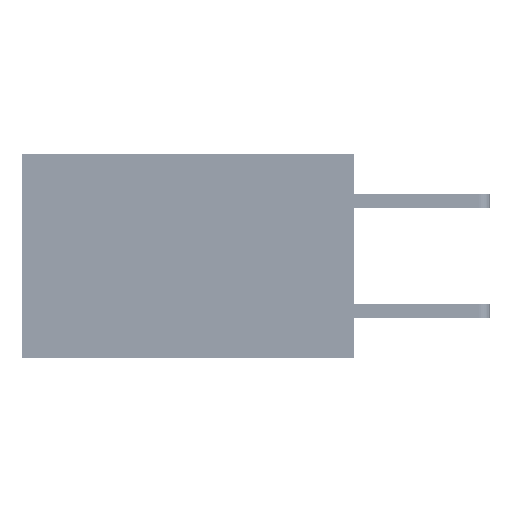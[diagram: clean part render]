
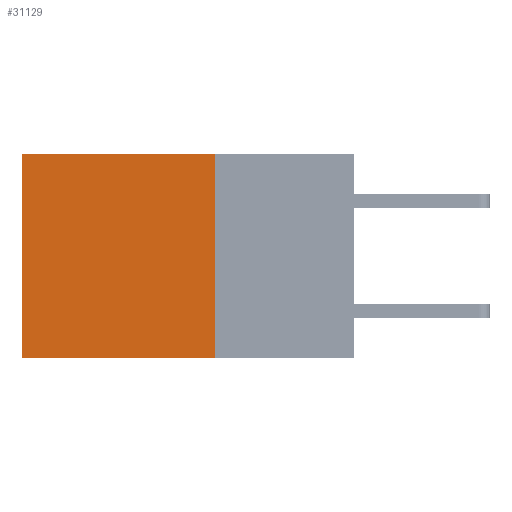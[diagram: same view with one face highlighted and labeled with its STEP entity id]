
A CAD part, left-side view. The second image highlights one B-rep face of the part: STEP entity #31129.
In plain terms, the highlighted planar face has unit normal (-1, 0, 0).
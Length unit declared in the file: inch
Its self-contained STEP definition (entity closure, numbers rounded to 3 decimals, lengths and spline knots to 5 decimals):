
#746 = LINE ( 'NONE', #25902, #8799 ) ;
#1346 = CARTESIAN_POINT ( 'NONE',  ( 0.2875, 0.25, -0.37 ) ) ;
#1725 = CARTESIAN_POINT ( 'NONE',  ( 0.2875, 0.6, 0. ) ) ;
#1906 = EDGE_CURVE ( 'NONE', #15443, #36825, #746, .T. ) ;
#3800 = DIRECTION ( 'NONE',  ( 0., 1., 0. ) ) ;
#3840 = LINE ( 'NONE', #25260, #8826 ) ;
#4311 = DIRECTION ( 'NONE',  ( 0., 0., -1. ) ) ;
#5148 = EDGE_CURVE ( 'NONE', #11501, #36459, #28958, .T. ) ;
#5820 = ORIENTED_EDGE ( 'NONE', *, *, #22225, .F. ) ;
#7561 = CARTESIAN_POINT ( 'NONE',  ( 0.2875, 0.25, 0. ) ) ;
#8109 = DIRECTION ( 'NONE',  ( 0., 0., -1. ) ) ;
#8799 = VECTOR ( 'NONE', #39999, 39.37008 ) ;
#8826 = VECTOR ( 'NONE', #4311, 39.37008 ) ;
#11277 = EDGE_CURVE ( 'NONE', #36459, #36825, #26444, .T. ) ;
#11501 = VERTEX_POINT ( 'NONE', #41472 ) ;
#15443 = VERTEX_POINT ( 'NONE', #1346 ) ;
#20829 = EDGE_LOOP ( 'NONE', ( #40693, #21456, #5820, #35009 ) ) ;
#21456 = ORIENTED_EDGE ( 'NONE', *, *, #1906, .F. ) ;
#21593 = AXIS2_PLACEMENT_3D ( 'NONE', #30158, #40530, #40075 ) ;
#22225 = EDGE_CURVE ( 'NONE', #11501, #15443, #3840, .T. ) ;
#25260 = CARTESIAN_POINT ( 'NONE',  ( 0.2875, 0.25, 0. ) ) ;
#25902 = CARTESIAN_POINT ( 'NONE',  ( 0.2875, 0.25, -0.37 ) ) ;
#26204 = PLANE ( 'NONE',  #21593 ) ;
#26444 = LINE ( 'NONE', #1725, #38294 ) ;
#28958 = LINE ( 'NONE', #7561, #40877 ) ;
#29705 = FACE_OUTER_BOUND ( 'NONE', #20829, .T. ) ;
#30158 = CARTESIAN_POINT ( 'NONE',  ( 0.2875, 0.25, 0. ) ) ;
#31129 = ADVANCED_FACE ( 'NONE', ( #29705 ), #26204, .F. ) ;
#35009 = ORIENTED_EDGE ( 'NONE', *, *, #5148, .T. ) ;
#36459 = VERTEX_POINT ( 'NONE', #43972 ) ;
#36825 = VERTEX_POINT ( 'NONE', #42766 ) ;
#38294 = VECTOR ( 'NONE', #8109, 39.37008 ) ;
#39999 = DIRECTION ( 'NONE',  ( 0., 1., 0. ) ) ;
#40075 = DIRECTION ( 'NONE',  ( 0., 0., -1. ) ) ;
#40530 = DIRECTION ( 'NONE',  ( 1., 0., 0. ) ) ;
#40693 = ORIENTED_EDGE ( 'NONE', *, *, #11277, .T. ) ;
#40877 = VECTOR ( 'NONE', #3800, 39.37008 ) ;
#41472 = CARTESIAN_POINT ( 'NONE',  ( 0.2875, 0.25, 0. ) ) ;
#42766 = CARTESIAN_POINT ( 'NONE',  ( 0.2875, 0.6, -0.37 ) ) ;
#43972 = CARTESIAN_POINT ( 'NONE',  ( 0.2875, 0.6, 0. ) ) ;
